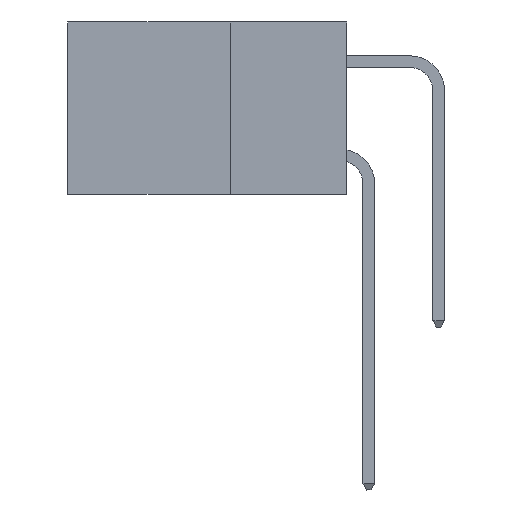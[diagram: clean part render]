
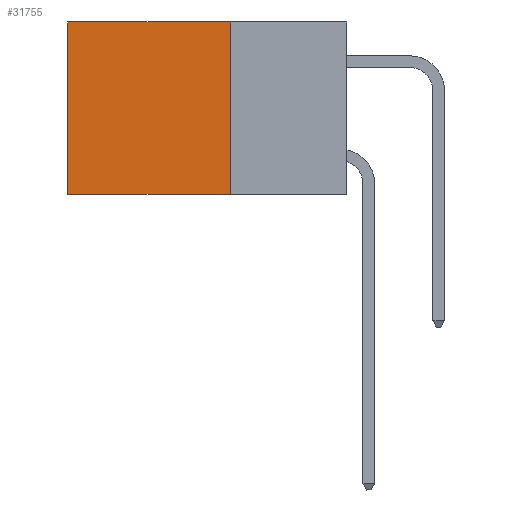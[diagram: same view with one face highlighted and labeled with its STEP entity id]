
A CAD part, left-side view. The second image highlights one B-rep face of the part: STEP entity #31755.
In plain terms, the highlighted planar face has unit normal (-1, 0, 0).
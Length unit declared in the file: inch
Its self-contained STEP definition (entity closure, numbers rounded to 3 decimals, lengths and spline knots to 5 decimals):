
#906 = ORIENTED_EDGE ( 'NONE', *, *, #6626, .T. ) ;
#1174 = CARTESIAN_POINT ( 'NONE',  ( 0.2875, 0.25, 0. ) ) ;
#1230 = CARTESIAN_POINT ( 'NONE',  ( 0.2875, 0.25, 0. ) ) ;
#4008 = VECTOR ( 'NONE', #18425, 39.37008 ) ;
#4807 = VERTEX_POINT ( 'NONE', #9950 ) ;
#5549 = EDGE_CURVE ( 'NONE', #13037, #22550, #21282, .T. ) ;
#6202 = DIRECTION ( 'NONE',  ( 1., 0., 0. ) ) ;
#6626 = EDGE_CURVE ( 'NONE', #4807, #24477, #12691, .T. ) ;
#7647 = EDGE_CURVE ( 'NONE', #24477, #22550, #31167, .T. ) ;
#9862 = DIRECTION ( 'NONE',  ( 0., 0., -1. ) ) ;
#9950 = CARTESIAN_POINT ( 'NONE',  ( 0.2875, 0.25, 0. ) ) ;
#10600 = ORIENTED_EDGE ( 'NONE', *, *, #7647, .T. ) ;
#11230 = DIRECTION ( 'NONE',  ( 0., 1., 0. ) ) ;
#12691 = LINE ( 'NONE', #1230, #17326 ) ;
#13037 = VERTEX_POINT ( 'NONE', #28520 ) ;
#13441 = DIRECTION ( 'NONE',  ( 0., 0., -1. ) ) ;
#14700 = VECTOR ( 'NONE', #24735, 39.37008 ) ;
#14854 = CARTESIAN_POINT ( 'NONE',  ( 0.2875, 0.25, -0.37 ) ) ;
#16358 = LINE ( 'NONE', #27732, #4008 ) ;
#17326 = VECTOR ( 'NONE', #11230, 39.37008 ) ;
#18425 = DIRECTION ( 'NONE',  ( 0., 0., -1. ) ) ;
#18797 = ORIENTED_EDGE ( 'NONE', *, *, #19021, .F. ) ;
#19021 = EDGE_CURVE ( 'NONE', #4807, #13037, #16358, .T. ) ;
#19309 = ORIENTED_EDGE ( 'NONE', *, *, #5549, .F. ) ;
#20971 = PLANE ( 'NONE',  #23531 ) ;
#21282 = LINE ( 'NONE', #14854, #14700 ) ;
#21337 = CARTESIAN_POINT ( 'NONE',  ( 0.2875, 0.6, 0. ) ) ;
#22550 = VERTEX_POINT ( 'NONE', #24272 ) ;
#23531 = AXIS2_PLACEMENT_3D ( 'NONE', #1174, #6202, #13441 ) ;
#24272 = CARTESIAN_POINT ( 'NONE',  ( 0.2875, 0.6, -0.37 ) ) ;
#24477 = VERTEX_POINT ( 'NONE', #21337 ) ;
#24735 = DIRECTION ( 'NONE',  ( 0., 1., 0. ) ) ;
#27385 = CARTESIAN_POINT ( 'NONE',  ( 0.2875, 0.6, 0. ) ) ;
#27732 = CARTESIAN_POINT ( 'NONE',  ( 0.2875, 0.25, 0. ) ) ;
#28520 = CARTESIAN_POINT ( 'NONE',  ( 0.2875, 0.25, -0.37 ) ) ;
#29939 = EDGE_LOOP ( 'NONE', ( #10600, #19309, #18797, #906 ) ) ;
#30064 = FACE_OUTER_BOUND ( 'NONE', #29939, .T. ) ;
#31167 = LINE ( 'NONE', #27385, #31570 ) ;
#31570 = VECTOR ( 'NONE', #9862, 39.37008 ) ;
#31755 = ADVANCED_FACE ( 'NONE', ( #30064 ), #20971, .F. ) ;
